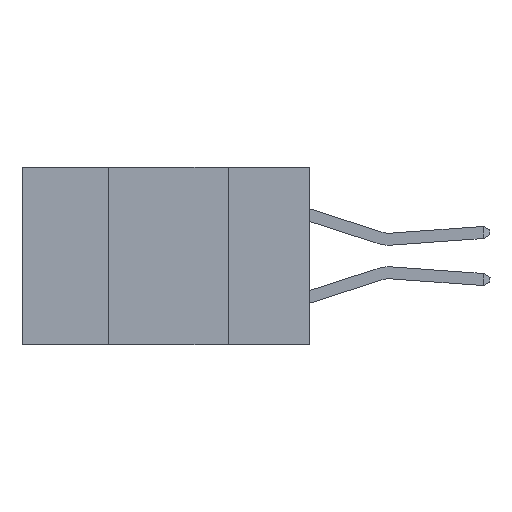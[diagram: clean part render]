
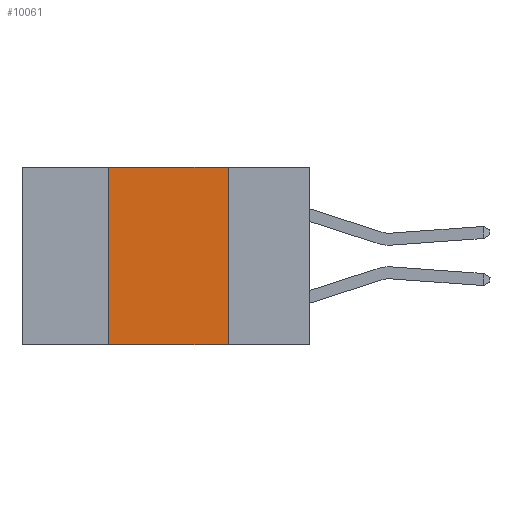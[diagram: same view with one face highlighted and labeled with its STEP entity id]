
A CAD part, left-side view. The second image highlights one B-rep face of the part: STEP entity #10061.
In plain terms, the highlighted planar face has unit normal (-1, 0, 0).
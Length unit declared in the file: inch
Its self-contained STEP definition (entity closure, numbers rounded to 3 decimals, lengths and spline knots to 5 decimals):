
#177 = CARTESIAN_POINT ( 'NONE',  ( 0., 0.42, -0.37 ) ) ;
#226 = ORIENTED_EDGE ( 'NONE', *, *, #19936, .T. ) ;
#600 = CARTESIAN_POINT ( 'NONE',  ( 0., 0.6, 0. ) ) ;
#669 = AXIS2_PLACEMENT_3D ( 'NONE', #600, #2164, #13136 ) ;
#780 = DIRECTION ( 'NONE',  ( 0., 0., 1. ) ) ;
#1177 = FACE_OUTER_BOUND ( 'NONE', #1350, .T. ) ;
#1350 = EDGE_LOOP ( 'NONE', ( #9944, #6422, #4675, #226 ) ) ;
#1489 = VECTOR ( 'NONE', #780, 39.37008 ) ;
#1654 = VERTEX_POINT ( 'NONE', #10506 ) ;
#2164 = DIRECTION ( 'NONE',  ( 1., 0., 0. ) ) ;
#3761 = VECTOR ( 'NONE', #15515, 39.37008 ) ;
#4656 = CARTESIAN_POINT ( 'NONE',  ( 0., 0.6, -0.37 ) ) ;
#4675 = ORIENTED_EDGE ( 'NONE', *, *, #14867, .F. ) ;
#6422 = ORIENTED_EDGE ( 'NONE', *, *, #16893, .F. ) ;
#6859 = CARTESIAN_POINT ( 'NONE',  ( 0., 0.17, -0.37 ) ) ;
#8111 = LINE ( 'NONE', #16609, #19831 ) ;
#9944 = ORIENTED_EDGE ( 'NONE', *, *, #12830, .F. ) ;
#10010 = PLANE ( 'NONE',  #669 ) ;
#10061 = ADVANCED_FACE ( 'NONE', ( #1177 ), #10010, .F. ) ;
#10325 = CARTESIAN_POINT ( 'NONE',  ( 0., 0.17, 0. ) ) ;
#10506 = CARTESIAN_POINT ( 'NONE',  ( 0., 0.42, 0. ) ) ;
#10675 = VERTEX_POINT ( 'NONE', #11401 ) ;
#11401 = CARTESIAN_POINT ( 'NONE',  ( 0., 0.17, -0.37 ) ) ;
#12241 = VERTEX_POINT ( 'NONE', #10325 ) ;
#12830 = EDGE_CURVE ( 'NONE', #12241, #10675, #18802, .T. ) ;
#13136 = DIRECTION ( 'NONE',  ( 0., 0., -1. ) ) ;
#13253 = CARTESIAN_POINT ( 'NONE',  ( 0., 0.42, -0.37 ) ) ;
#14775 = VECTOR ( 'NONE', #19149, 39.37008 ) ;
#14867 = EDGE_CURVE ( 'NONE', #16497, #1654, #18020, .T. ) ;
#15515 = DIRECTION ( 'NONE',  ( 0., -1., 0. ) ) ;
#16497 = VERTEX_POINT ( 'NONE', #177 ) ;
#16549 = DIRECTION ( 'NONE',  ( 0., -1., 0. ) ) ;
#16609 = CARTESIAN_POINT ( 'NONE',  ( 0., 0.6, 0. ) ) ;
#16893 = EDGE_CURVE ( 'NONE', #1654, #12241, #8111, .T. ) ;
#18020 = LINE ( 'NONE', #13253, #1489 ) ;
#18802 = LINE ( 'NONE', #6859, #14775 ) ;
#19149 = DIRECTION ( 'NONE',  ( 0., 0., -1. ) ) ;
#19691 = LINE ( 'NONE', #4656, #3761 ) ;
#19831 = VECTOR ( 'NONE', #16549, 39.37008 ) ;
#19936 = EDGE_CURVE ( 'NONE', #16497, #10675, #19691, .T. ) ;
